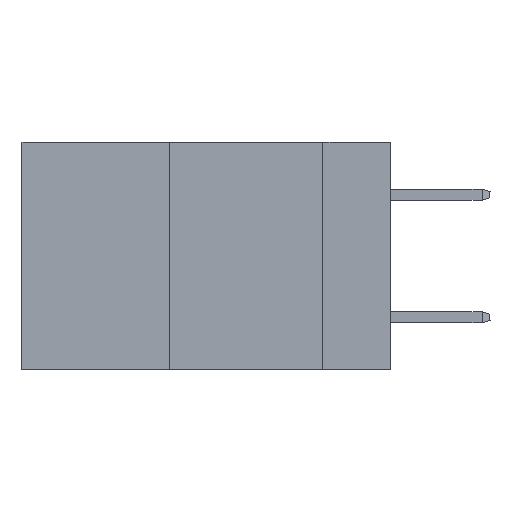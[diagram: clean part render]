
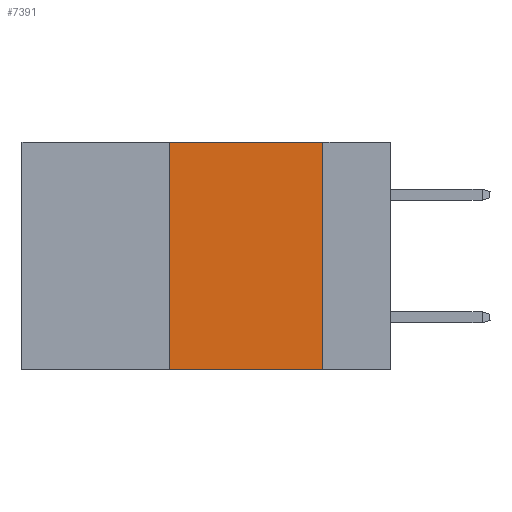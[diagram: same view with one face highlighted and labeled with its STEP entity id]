
A CAD part, left-side view. The second image highlights one B-rep face of the part: STEP entity #7391.
In plain terms, the highlighted planar face has unit normal (-1, 0, 0).
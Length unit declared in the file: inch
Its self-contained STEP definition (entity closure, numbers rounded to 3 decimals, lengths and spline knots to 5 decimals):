
#845 = VECTOR ( 'NONE', #14813, 39.37008 ) ;
#6193 = VERTEX_POINT ( 'NONE', #31916 ) ;
#6723 = ORIENTED_EDGE ( 'NONE', *, *, #30568, .T. ) ;
#7391 = ADVANCED_FACE ( 'NONE', ( #41333 ), #10578, .F. ) ;
#8548 = VERTEX_POINT ( 'NONE', #37098 ) ;
#8772 = VECTOR ( 'NONE', #34665, 39.37008 ) ;
#9327 = LINE ( 'NONE', #24198, #8772 ) ;
#10578 = PLANE ( 'NONE',  #19830 ) ;
#14566 = CARTESIAN_POINT ( 'NONE',  ( 0., 0.6, -0.37 ) ) ;
#14813 = DIRECTION ( 'NONE',  ( 0., 0., 1. ) ) ;
#17689 = DIRECTION ( 'NONE',  ( 0., 0., -1. ) ) ;
#18222 = DIRECTION ( 'NONE',  ( 0., -1., 0. ) ) ;
#19267 = VERTEX_POINT ( 'NONE', #42168 ) ;
#19830 = AXIS2_PLACEMENT_3D ( 'NONE', #39357, #42985, #17689 ) ;
#24198 = CARTESIAN_POINT ( 'NONE',  ( 0., 0.11, 0. ) ) ;
#24790 = LINE ( 'NONE', #46814, #40615 ) ;
#25121 = ORIENTED_EDGE ( 'NONE', *, *, #41486, .F. ) ;
#26640 = EDGE_CURVE ( 'NONE', #19267, #36128, #39892, .T. ) ;
#29758 = ORIENTED_EDGE ( 'NONE', *, *, #37793, .F. ) ;
#30568 = EDGE_CURVE ( 'NONE', #19267, #8548, #43079, .T. ) ;
#31916 = CARTESIAN_POINT ( 'NONE',  ( 0., 0.11, 0. ) ) ;
#31926 = ORIENTED_EDGE ( 'NONE', *, *, #26640, .F. ) ;
#32149 = DIRECTION ( 'NONE',  ( 0., -1., 0. ) ) ;
#33365 = CARTESIAN_POINT ( 'NONE',  ( 0., 0.36, 0. ) ) ;
#34622 = VECTOR ( 'NONE', #18222, 39.37008 ) ;
#34665 = DIRECTION ( 'NONE',  ( 0., 0., -1. ) ) ;
#34821 = EDGE_LOOP ( 'NONE', ( #29758, #25121, #31926, #6723 ) ) ;
#36128 = VERTEX_POINT ( 'NONE', #45672 ) ;
#37098 = CARTESIAN_POINT ( 'NONE',  ( 0., 0.11, -0.37 ) ) ;
#37793 = EDGE_CURVE ( 'NONE', #6193, #8548, #9327, .T. ) ;
#39357 = CARTESIAN_POINT ( 'NONE',  ( 0., 0.6, 0. ) ) ;
#39892 = LINE ( 'NONE', #33365, #845 ) ;
#40615 = VECTOR ( 'NONE', #32149, 39.37008 ) ;
#41333 = FACE_OUTER_BOUND ( 'NONE', #34821, .T. ) ;
#41486 = EDGE_CURVE ( 'NONE', #36128, #6193, #24790, .T. ) ;
#42168 = CARTESIAN_POINT ( 'NONE',  ( 0., 0.36, -0.37 ) ) ;
#42985 = DIRECTION ( 'NONE',  ( 1., 0., 0. ) ) ;
#43079 = LINE ( 'NONE', #14566, #34622 ) ;
#45672 = CARTESIAN_POINT ( 'NONE',  ( 0., 0.36, 0. ) ) ;
#46814 = CARTESIAN_POINT ( 'NONE',  ( 0., 0.6, 0. ) ) ;
